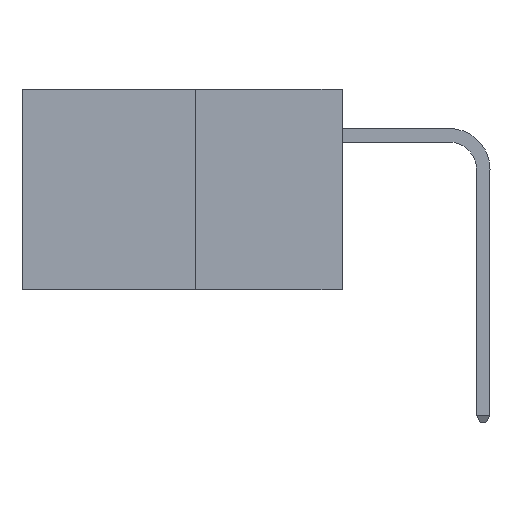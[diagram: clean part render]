
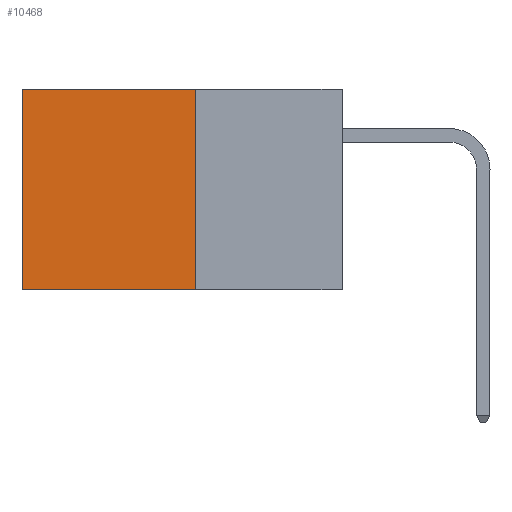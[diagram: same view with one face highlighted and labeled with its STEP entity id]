
A CAD part, left-side view. The second image highlights one B-rep face of the part: STEP entity #10468.
In plain terms, the highlighted planar face has unit normal (-1, 0, 0).
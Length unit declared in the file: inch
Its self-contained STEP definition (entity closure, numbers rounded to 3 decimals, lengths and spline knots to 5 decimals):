
#106 = DIRECTION ( 'NONE',  ( 0., 1., 0. ) ) ;
#548 = CARTESIAN_POINT ( 'NONE',  ( 0.277, 0.27, -0.37 ) ) ;
#713 = FACE_OUTER_BOUND ( 'NONE', #972, .T. ) ;
#795 = LINE ( 'NONE', #12747, #4906 ) ;
#972 = EDGE_LOOP ( 'NONE', ( #5490, #12024, #16803, #4360 ) ) ;
#1048 = CARTESIAN_POINT ( 'NONE',  ( 0.277, 0.27, -0.37 ) ) ;
#2331 = CARTESIAN_POINT ( 'NONE',  ( 0.277, 0.27, -0.37 ) ) ;
#2485 = VECTOR ( 'NONE', #14416, 39.37008 ) ;
#3067 = CARTESIAN_POINT ( 'NONE',  ( 0.277, 0.59, -0.37 ) ) ;
#3596 = DIRECTION ( 'NONE',  ( 0., 0., -1. ) ) ;
#3684 = VERTEX_POINT ( 'NONE', #14049 ) ;
#3874 = DIRECTION ( 'NONE',  ( 0., 1., 0. ) ) ;
#4360 = ORIENTED_EDGE ( 'NONE', *, *, #15466, .T. ) ;
#4564 = CARTESIAN_POINT ( 'NONE',  ( 0.277, 0.59, 0. ) ) ;
#4906 = VECTOR ( 'NONE', #3596, 39.37008 ) ;
#5490 = ORIENTED_EDGE ( 'NONE', *, *, #6988, .T. ) ;
#6875 = CARTESIAN_POINT ( 'NONE',  ( 0.277, 0.59, -0.37 ) ) ;
#6988 = EDGE_CURVE ( 'NONE', #18362, #12999, #18537, .T. ) ;
#8296 = PLANE ( 'NONE',  #17137 ) ;
#8326 = VERTEX_POINT ( 'NONE', #1048 ) ;
#8364 = VECTOR ( 'NONE', #3874, 39.37008 ) ;
#8731 = EDGE_CURVE ( 'NONE', #3684, #8326, #795, .T. ) ;
#9815 = DIRECTION ( 'NONE',  ( 0., 0., -1. ) ) ;
#10468 = ADVANCED_FACE ( 'NONE', ( #713 ), #8296, .F. ) ;
#11827 = EDGE_CURVE ( 'NONE', #8326, #12999, #15861, .T. ) ;
#11899 = LINE ( 'NONE', #16818, #14889 ) ;
#12024 = ORIENTED_EDGE ( 'NONE', *, *, #11827, .F. ) ;
#12747 = CARTESIAN_POINT ( 'NONE',  ( 0.277, 0.27, -0.37 ) ) ;
#12999 = VERTEX_POINT ( 'NONE', #3067 ) ;
#14049 = CARTESIAN_POINT ( 'NONE',  ( 0.277, 0.27, 0. ) ) ;
#14416 = DIRECTION ( 'NONE',  ( 0., 0., -1. ) ) ;
#14889 = VECTOR ( 'NONE', #106, 39.37008 ) ;
#15466 = EDGE_CURVE ( 'NONE', #3684, #18362, #11899, .T. ) ;
#15861 = LINE ( 'NONE', #2331, #8364 ) ;
#16803 = ORIENTED_EDGE ( 'NONE', *, *, #8731, .F. ) ;
#16818 = CARTESIAN_POINT ( 'NONE',  ( 0.277, 0.27, 0. ) ) ;
#17137 = AXIS2_PLACEMENT_3D ( 'NONE', #548, #18750, #9815 ) ;
#18362 = VERTEX_POINT ( 'NONE', #4564 ) ;
#18537 = LINE ( 'NONE', #6875, #2485 ) ;
#18750 = DIRECTION ( 'NONE',  ( 1., 0., 0. ) ) ;
